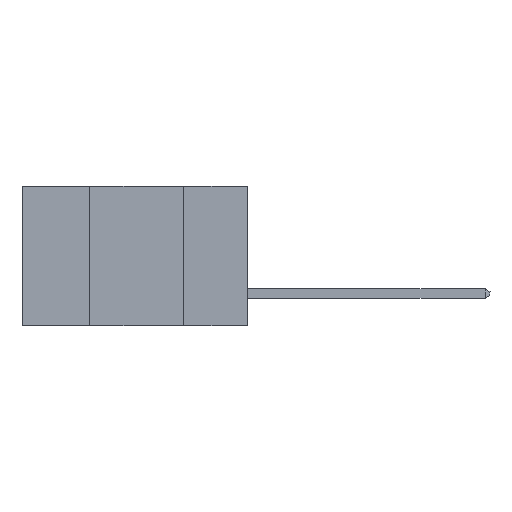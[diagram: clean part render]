
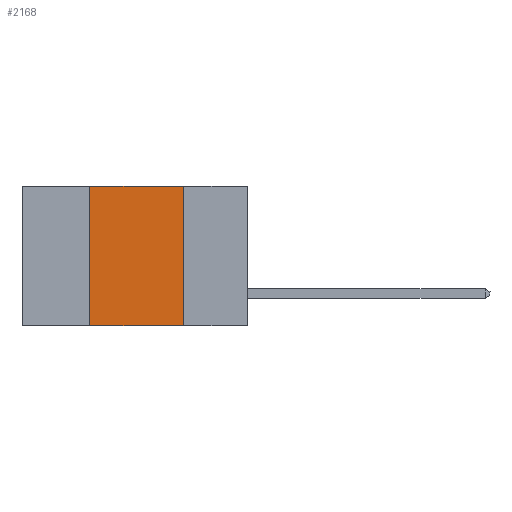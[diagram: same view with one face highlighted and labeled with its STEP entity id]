
A CAD part, left-side view. The second image highlights one B-rep face of the part: STEP entity #2168.
In plain terms, the highlighted planar face has unit normal (-1, 0, 0).
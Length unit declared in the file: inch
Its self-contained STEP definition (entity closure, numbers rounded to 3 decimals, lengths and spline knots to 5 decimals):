
#130 = CARTESIAN_POINT ( 'NONE',  ( 0., 0.42, -0.37 ) ) ;
#830 = DIRECTION ( 'NONE',  ( 0., 0., -1. ) ) ;
#899 = LINE ( 'NONE', #130, #3349 ) ;
#1014 = VECTOR ( 'NONE', #830, 39.37008 ) ;
#1266 = LINE ( 'NONE', #9796, #7000 ) ;
#1793 = VERTEX_POINT ( 'NONE', #8248 ) ;
#1828 = FACE_OUTER_BOUND ( 'NONE', #7275, .T. ) ;
#1875 = DIRECTION ( 'NONE',  ( 0., -1., 0. ) ) ;
#1915 = CARTESIAN_POINT ( 'NONE',  ( 0., 0.17, 0. ) ) ;
#1923 = CARTESIAN_POINT ( 'NONE',  ( 0., 0.6, 0. ) ) ;
#2168 = ADVANCED_FACE ( 'NONE', ( #1828 ), #3443, .F. ) ;
#2463 = DIRECTION ( 'NONE',  ( 0., 0., 1. ) ) ;
#3154 = LINE ( 'NONE', #6109, #1014 ) ;
#3349 = VECTOR ( 'NONE', #2463, 39.37008 ) ;
#3439 = ORIENTED_EDGE ( 'NONE', *, *, #7912, .T. ) ;
#3443 = PLANE ( 'NONE',  #9902 ) ;
#3568 = CARTESIAN_POINT ( 'NONE',  ( 0., 0.42, -0.37 ) ) ;
#5133 = VERTEX_POINT ( 'NONE', #3568 ) ;
#5361 = EDGE_CURVE ( 'NONE', #5133, #1793, #899, .T. ) ;
#5814 = ORIENTED_EDGE ( 'NONE', *, *, #8774, .F. ) ;
#6008 = CARTESIAN_POINT ( 'NONE',  ( 0., 0.17, -0.37 ) ) ;
#6109 = CARTESIAN_POINT ( 'NONE',  ( 0., 0.17, -0.37 ) ) ;
#6475 = CARTESIAN_POINT ( 'NONE',  ( 0., 0.6, 0. ) ) ;
#6584 = VERTEX_POINT ( 'NONE', #6008 ) ;
#7000 = VECTOR ( 'NONE', #7388, 39.37008 ) ;
#7275 = EDGE_LOOP ( 'NONE', ( #8735, #5814, #8220, #3439 ) ) ;
#7388 = DIRECTION ( 'NONE',  ( 0., -1., 0. ) ) ;
#7730 = VERTEX_POINT ( 'NONE', #1915 ) ;
#7912 = EDGE_CURVE ( 'NONE', #5133, #6584, #1266, .T. ) ;
#7943 = VECTOR ( 'NONE', #1875, 39.37008 ) ;
#7948 = DIRECTION ( 'NONE',  ( 0., 0., -1. ) ) ;
#8007 = DIRECTION ( 'NONE',  ( 1., 0., 0. ) ) ;
#8048 = LINE ( 'NONE', #1923, #7943 ) ;
#8220 = ORIENTED_EDGE ( 'NONE', *, *, #5361, .F. ) ;
#8248 = CARTESIAN_POINT ( 'NONE',  ( 0., 0.42, 0. ) ) ;
#8735 = ORIENTED_EDGE ( 'NONE', *, *, #9890, .F. ) ;
#8774 = EDGE_CURVE ( 'NONE', #1793, #7730, #8048, .T. ) ;
#9796 = CARTESIAN_POINT ( 'NONE',  ( 0., 0.6, -0.37 ) ) ;
#9890 = EDGE_CURVE ( 'NONE', #7730, #6584, #3154, .T. ) ;
#9902 = AXIS2_PLACEMENT_3D ( 'NONE', #6475, #8007, #7948 ) ;
